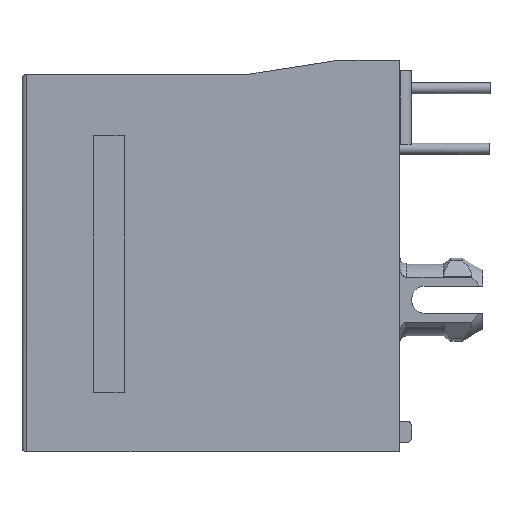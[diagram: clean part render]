
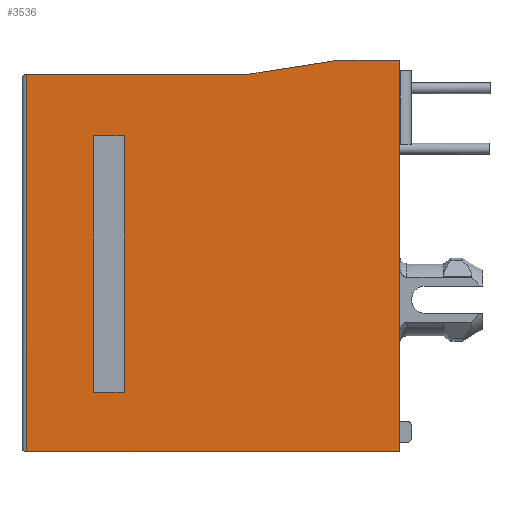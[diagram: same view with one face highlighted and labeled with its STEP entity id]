
A CAD part, left-side view. The second image highlights one B-rep face of the part: STEP entity #3536.
In plain terms, the highlighted planar face has unit normal (-1, 0, 0).
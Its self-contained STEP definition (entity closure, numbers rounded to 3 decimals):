
#42 = DIRECTION ( 'NONE',  ( 0., -0.988, 0.154 ) ) ;
#77 = LINE ( 'NONE', #4623, #2066 ) ;
#339 = VECTOR ( 'NONE', #7323, 1000. ) ;
#388 = ORIENTED_EDGE ( 'NONE', *, *, #402, .F. ) ;
#402 = EDGE_CURVE ( 'NONE', #6745, #5184, #562, .T. ) ;
#562 = LINE ( 'NONE', #3674, #6596 ) ;
#763 = VECTOR ( 'NONE', #7017, 1000. ) ;
#785 = VECTOR ( 'NONE', #9287, 1000. ) ;
#801 = CARTESIAN_POINT ( 'NONE',  ( -5.75, -7.94, -0.829 ) ) ;
#1125 = CARTESIAN_POINT ( 'NONE',  ( -5.75, 4.94, 12.471 ) ) ;
#1235 = VERTEX_POINT ( 'NONE', #5046 ) ;
#1511 = DIRECTION ( 'NONE',  ( 0., 0., -1. ) ) ;
#1519 = ORIENTED_EDGE ( 'NONE', *, *, #8120, .F. ) ;
#1586 = DIRECTION ( 'NONE',  ( 0., 0., 1. ) ) ;
#1668 = EDGE_CURVE ( 'NONE', #5184, #8032, #11545, .T. ) ;
#1853 = PLANE ( 'NONE',  #3157 ) ;
#2066 = VECTOR ( 'NONE', #7347, 1000. ) ;
#2088 = EDGE_CURVE ( 'NONE', #4576, #1235, #10975, .T. ) ;
#2241 = VECTOR ( 'NONE', #3478, 1000. ) ;
#2291 = ORIENTED_EDGE ( 'NONE', *, *, #2088, .F. ) ;
#3157 = AXIS2_PLACEMENT_3D ( 'NONE', #3619, #8157, #5381 ) ;
#3478 = DIRECTION ( 'NONE',  ( 0., 1., 0. ) ) ;
#3500 = EDGE_CURVE ( 'NONE', #1235, #10870, #6660, .T. ) ;
#3536 = ADVANCED_FACE ( 'NONE', ( #7082, #8940 ), #1853, .F. ) ;
#3619 = CARTESIAN_POINT ( 'NONE',  ( -5.75, -7.94, 15.651 ) ) ;
#3657 = ORIENTED_EDGE ( 'NONE', *, *, #3500, .F. ) ;
#3674 = CARTESIAN_POINT ( 'NONE',  ( -5.75, -5.42, 15.651 ) ) ;
#4157 = CARTESIAN_POINT ( 'NONE',  ( -5.75, 4.94, 1.671 ) ) ;
#4576 = VERTEX_POINT ( 'NONE', #4157 ) ;
#4620 = LINE ( 'NONE', #801, #2241 ) ;
#4623 = CARTESIAN_POINT ( 'NONE',  ( -5.75, 4.94, 15.651 ) ) ;
#4926 = VERTEX_POINT ( 'NONE', #11736 ) ;
#4976 = CARTESIAN_POINT ( 'NONE',  ( -5.75, 7.74, -0.829 ) ) ;
#5046 = CARTESIAN_POINT ( 'NONE',  ( -5.75, 3.64, 1.671 ) ) ;
#5176 = CARTESIAN_POINT ( 'NONE',  ( -5.75, -1.56, 15.051 ) ) ;
#5184 = VERTEX_POINT ( 'NONE', #5990 ) ;
#5211 = EDGE_LOOP ( 'NONE', ( #2291, #1519, #11628, #3657 ) ) ;
#5329 = CARTESIAN_POINT ( 'NONE',  ( -5.75, -7.94, -0.829 ) ) ;
#5381 = DIRECTION ( 'NONE',  ( 0., -1., 0. ) ) ;
#5494 = CARTESIAN_POINT ( 'NONE',  ( -5.75, 7.74, 15.651 ) ) ;
#5582 = EDGE_CURVE ( 'NONE', #10870, #7832, #9610, .T. ) ;
#5809 = CARTESIAN_POINT ( 'NONE',  ( -5.75, 3.64, 12.471 ) ) ;
#5955 = CARTESIAN_POINT ( 'NONE',  ( -5.75, -7.94, 15.051 ) ) ;
#5990 = CARTESIAN_POINT ( 'NONE',  ( -5.75, -7.94, 15.651 ) ) ;
#6165 = VECTOR ( 'NONE', #42, 1000. ) ;
#6197 = EDGE_CURVE ( 'NONE', #8032, #7935, #4620, .T. ) ;
#6242 = ORIENTED_EDGE ( 'NONE', *, *, #6250, .F. ) ;
#6250 = EDGE_CURVE ( 'NONE', #4926, #6745, #10016, .T. ) ;
#6596 = VECTOR ( 'NONE', #9265, 1000. ) ;
#6660 = LINE ( 'NONE', #9816, #11368 ) ;
#6745 = VERTEX_POINT ( 'NONE', #9753 ) ;
#6793 = ORIENTED_EDGE ( 'NONE', *, *, #6197, .F. ) ;
#7017 = DIRECTION ( 'NONE',  ( 0., -1., 0. ) ) ;
#7082 = FACE_BOUND ( 'NONE', #5211, .T. ) ;
#7323 = DIRECTION ( 'NONE',  ( 0., 0., 1. ) ) ;
#7347 = DIRECTION ( 'NONE',  ( 0., 0., -1. ) ) ;
#7555 = ORIENTED_EDGE ( 'NONE', *, *, #9361, .F. ) ;
#7832 = VERTEX_POINT ( 'NONE', #1125 ) ;
#7935 = VERTEX_POINT ( 'NONE', #4976 ) ;
#8032 = VERTEX_POINT ( 'NONE', #5329 ) ;
#8120 = EDGE_CURVE ( 'NONE', #7832, #4576, #77, .T. ) ;
#8157 = DIRECTION ( 'NONE',  ( 1., 0., 0. ) ) ;
#8359 = CARTESIAN_POINT ( 'NONE',  ( -5.75, -7.94, 1.671 ) ) ;
#8375 = LINE ( 'NONE', #5494, #339 ) ;
#8829 = CARTESIAN_POINT ( 'NONE',  ( -5.75, -7.94, 12.471 ) ) ;
#8940 = FACE_OUTER_BOUND ( 'NONE', #10623, .T. ) ;
#9262 = VECTOR ( 'NONE', #1511, 1000. ) ;
#9265 = DIRECTION ( 'NONE',  ( 0., -1., 0. ) ) ;
#9287 = DIRECTION ( 'NONE',  ( 0., -1., 0. ) ) ;
#9361 = EDGE_CURVE ( 'NONE', #11222, #4926, #10093, .T. ) ;
#9592 = EDGE_CURVE ( 'NONE', #7935, #11222, #8375, .T. ) ;
#9610 = LINE ( 'NONE', #8829, #10175 ) ;
#9731 = CARTESIAN_POINT ( 'NONE',  ( -5.75, 7.74, 15.051 ) ) ;
#9753 = CARTESIAN_POINT ( 'NONE',  ( -5.75, -5.42, 15.651 ) ) ;
#9757 = DIRECTION ( 'NONE',  ( 0., 1., 0. ) ) ;
#9816 = CARTESIAN_POINT ( 'NONE',  ( -5.75, 3.64, 15.651 ) ) ;
#9900 = ORIENTED_EDGE ( 'NONE', *, *, #9592, .F. ) ;
#10016 = LINE ( 'NONE', #10951, #6165 ) ;
#10093 = LINE ( 'NONE', #5176, #763 ) ;
#10175 = VECTOR ( 'NONE', #9757, 1000. ) ;
#10623 = EDGE_LOOP ( 'NONE', ( #9900, #6793, #10973, #388, #6242, #7555 ) ) ;
#10870 = VERTEX_POINT ( 'NONE', #5809 ) ;
#10951 = CARTESIAN_POINT ( 'NONE',  ( -5.75, -1.56, 15.051 ) ) ;
#10973 = ORIENTED_EDGE ( 'NONE', *, *, #1668, .F. ) ;
#10975 = LINE ( 'NONE', #8359, #785 ) ;
#11222 = VERTEX_POINT ( 'NONE', #9731 ) ;
#11368 = VECTOR ( 'NONE', #1586, 1000. ) ;
#11545 = LINE ( 'NONE', #5955, #9262 ) ;
#11628 = ORIENTED_EDGE ( 'NONE', *, *, #5582, .F. ) ;
#11736 = CARTESIAN_POINT ( 'NONE',  ( -5.75, -1.56, 15.051 ) ) ;
